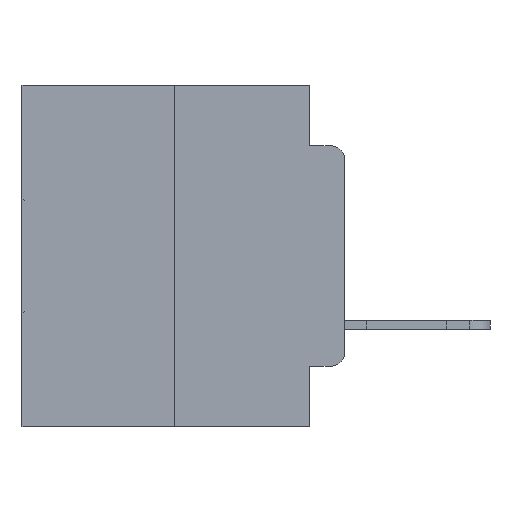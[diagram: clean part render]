
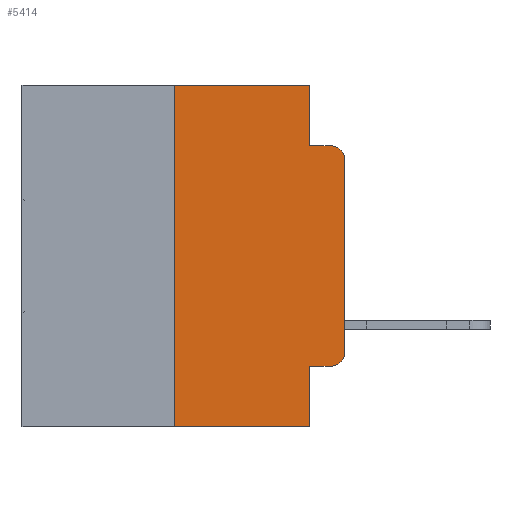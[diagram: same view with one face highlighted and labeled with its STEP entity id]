
A CAD part, left-side view. The second image highlights one B-rep face of the part: STEP entity #5414.
In plain terms, the highlighted planar face has unit normal (-1, 0, 0).
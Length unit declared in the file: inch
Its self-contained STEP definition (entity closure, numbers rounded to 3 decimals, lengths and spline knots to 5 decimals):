
#854 = LINE ( 'NONE', #27112, #25176 ) ;
#1030 = VECTOR ( 'NONE', #14290, 39.37008 ) ;
#1568 = LINE ( 'NONE', #29926, #8368 ) ;
#1772 = AXIS2_PLACEMENT_3D ( 'NONE', #5507, #6701, #28194 ) ;
#1885 = LINE ( 'NONE', #3905, #1030 ) ;
#2299 = DIRECTION ( 'NONE',  ( 0., 0., -1. ) ) ;
#2539 = CARTESIAN_POINT ( 'NONE',  ( 0., 0.051, 0. ) ) ;
#3198 = LINE ( 'NONE', #2539, #15493 ) ;
#3905 = CARTESIAN_POINT ( 'NONE',  ( 0., 0.473, -0.5 ) ) ;
#4890 = DIRECTION ( 'NONE',  ( -1., 0., 0. ) ) ;
#5303 = CARTESIAN_POINT ( 'NONE',  ( 0., 0., 0. ) ) ;
#5393 = DIRECTION ( 'NONE',  ( 0., 0., 1. ) ) ;
#5414 = ADVANCED_FACE ( 'NONE', ( #19277 ), #21746, .F. ) ;
#5507 = CARTESIAN_POINT ( 'NONE',  ( 0., 0.473, 0. ) ) ;
#5628 = LINE ( 'NONE', #26431, #18959 ) ;
#6701 = DIRECTION ( 'NONE',  ( 1., 0., 0. ) ) ;
#7548 = VERTEX_POINT ( 'NONE', #29055 ) ;
#8368 = VECTOR ( 'NONE', #29850, 39.37008 ) ;
#8388 = EDGE_CURVE ( 'NONE', #19150, #21285, #854, .T. ) ;
#9580 = LINE ( 'NONE', #5303, #15133 ) ;
#10544 = CARTESIAN_POINT ( 'NONE',  ( 0., 0.051, -0.0885 ) ) ;
#12451 = CARTESIAN_POINT ( 'NONE',  ( 0., 0.051, 0. ) ) ;
#12558 = CIRCLE ( 'NONE', #24212, 0.02 ) ;
#12712 = VERTEX_POINT ( 'NONE', #26640 ) ;
#13016 = VECTOR ( 'NONE', #13135, 39.37008 ) ;
#13135 = DIRECTION ( 'NONE',  ( 0., -1., 0. ) ) ;
#14290 = DIRECTION ( 'NONE',  ( 0., -1., 0. ) ) ;
#14514 = VERTEX_POINT ( 'NONE', #24454 ) ;
#15133 = VECTOR ( 'NONE', #5393, 39.37008 ) ;
#15493 = VECTOR ( 'NONE', #2299, 39.37008 ) ;
#17250 = DIRECTION ( 'NONE',  ( 0., 0., -1. ) ) ;
#17257 = DIRECTION ( 'NONE',  ( -1., 0., 0. ) ) ;
#17285 = CARTESIAN_POINT ( 'NONE',  ( 0., 0.02, -0.3915 ) ) ;
#17439 = VERTEX_POINT ( 'NONE', #28302 ) ;
#18010 = CIRCLE ( 'NONE', #27878, 0.02 ) ;
#18457 = DIRECTION ( 'NONE',  ( 0., 0., -1. ) ) ;
#18523 = CARTESIAN_POINT ( 'NONE',  ( 0., 0.02, -0.1085 ) ) ;
#18805 = EDGE_CURVE ( 'NONE', #12712, #21769, #1885, .T. ) ;
#18959 = VECTOR ( 'NONE', #26654, 39.37008 ) ;
#19150 = VERTEX_POINT ( 'NONE', #28097 ) ;
#19277 = FACE_OUTER_BOUND ( 'NONE', #22998, .T. ) ;
#19315 = VERTEX_POINT ( 'NONE', #24925 ) ;
#20779 = CARTESIAN_POINT ( 'NONE',  ( 0., 0.051, -0.4115 ) ) ;
#20883 = VECTOR ( 'NONE', #22600, 39.37008 ) ;
#21285 = VERTEX_POINT ( 'NONE', #12451 ) ;
#21579 = LINE ( 'NONE', #22770, #20883 ) ;
#21746 = PLANE ( 'NONE',  #1772 ) ;
#21769 = VERTEX_POINT ( 'NONE', #27189 ) ;
#21861 = VERTEX_POINT ( 'NONE', #20779 ) ;
#22439 = CARTESIAN_POINT ( 'NONE',  ( 0., 0.02, -0.4115 ) ) ;
#22600 = DIRECTION ( 'NONE',  ( 0., -1., 0. ) ) ;
#22770 = CARTESIAN_POINT ( 'NONE',  ( 0., 0.051, -0.4115 ) ) ;
#22998 = EDGE_LOOP ( 'NONE', ( #28084, #28138, #28234, #28324, #28375, #28538, #28748, #28903, #28954, #28994 ) ) ;
#23657 = EDGE_CURVE ( 'NONE', #19315, #14514, #9580, .T. ) ;
#24015 = EDGE_CURVE ( 'NONE', #14514, #17439, #18010, .T. ) ;
#24212 = AXIS2_PLACEMENT_3D ( 'NONE', #17285, #17257, #17250 ) ;
#24231 = EDGE_CURVE ( 'NONE', #7548, #17439, #24758, .T. ) ;
#24399 = EDGE_CURVE ( 'NONE', #21285, #7548, #3198, .T. ) ;
#24442 = EDGE_CURVE ( 'NONE', #12712, #19150, #1568, .T. ) ;
#24454 = CARTESIAN_POINT ( 'NONE',  ( 0., 0., -0.1085 ) ) ;
#24728 = EDGE_CURVE ( 'NONE', #21861, #21769, #5628, .T. ) ;
#24758 = LINE ( 'NONE', #10544, #13016 ) ;
#24925 = CARTESIAN_POINT ( 'NONE',  ( 0., 0., -0.3915 ) ) ;
#25019 = EDGE_CURVE ( 'NONE', #21861, #26870, #21579, .T. ) ;
#25176 = VECTOR ( 'NONE', #26770, 39.37008 ) ;
#25360 = EDGE_CURVE ( 'NONE', #26870, #19315, #12558, .T. ) ;
#26431 = CARTESIAN_POINT ( 'NONE',  ( 0., 0.051, 0. ) ) ;
#26640 = CARTESIAN_POINT ( 'NONE',  ( 0., 0.25, -0.5 ) ) ;
#26654 = DIRECTION ( 'NONE',  ( 0., 0., -1. ) ) ;
#26770 = DIRECTION ( 'NONE',  ( 0., -1., 0. ) ) ;
#26870 = VERTEX_POINT ( 'NONE', #22439 ) ;
#27112 = CARTESIAN_POINT ( 'NONE',  ( 0., 0.473, 0. ) ) ;
#27189 = CARTESIAN_POINT ( 'NONE',  ( 0., 0.051, -0.5 ) ) ;
#27878 = AXIS2_PLACEMENT_3D ( 'NONE', #18523, #4890, #18457 ) ;
#28084 = ORIENTED_EDGE ( 'NONE', *, *, #23657, .T. ) ;
#28097 = CARTESIAN_POINT ( 'NONE',  ( 0., 0.25, 0. ) ) ;
#28138 = ORIENTED_EDGE ( 'NONE', *, *, #24015, .T. ) ;
#28194 = DIRECTION ( 'NONE',  ( 0., 0., -1. ) ) ;
#28234 = ORIENTED_EDGE ( 'NONE', *, *, #24231, .F. ) ;
#28302 = CARTESIAN_POINT ( 'NONE',  ( 0., 0.02, -0.0885 ) ) ;
#28324 = ORIENTED_EDGE ( 'NONE', *, *, #24399, .F. ) ;
#28375 = ORIENTED_EDGE ( 'NONE', *, *, #8388, .F. ) ;
#28538 = ORIENTED_EDGE ( 'NONE', *, *, #24442, .F. ) ;
#28748 = ORIENTED_EDGE ( 'NONE', *, *, #18805, .T. ) ;
#28903 = ORIENTED_EDGE ( 'NONE', *, *, #24728, .F. ) ;
#28954 = ORIENTED_EDGE ( 'NONE', *, *, #25019, .T. ) ;
#28994 = ORIENTED_EDGE ( 'NONE', *, *, #25360, .T. ) ;
#29055 = CARTESIAN_POINT ( 'NONE',  ( 0., 0.051, -0.0885 ) ) ;
#29850 = DIRECTION ( 'NONE',  ( 0., 0., 1. ) ) ;
#29926 = CARTESIAN_POINT ( 'NONE',  ( 0., 0.25, 0. ) ) ;
